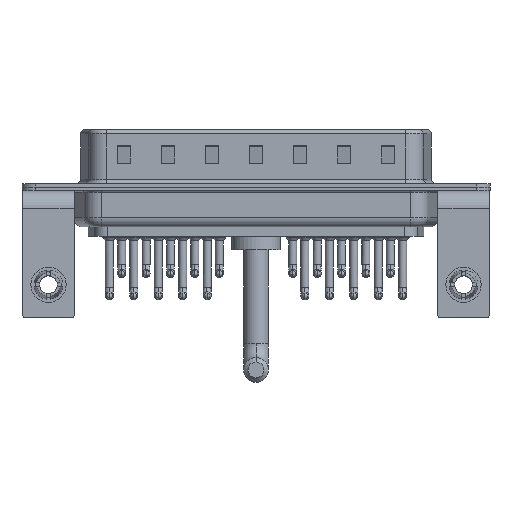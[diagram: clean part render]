
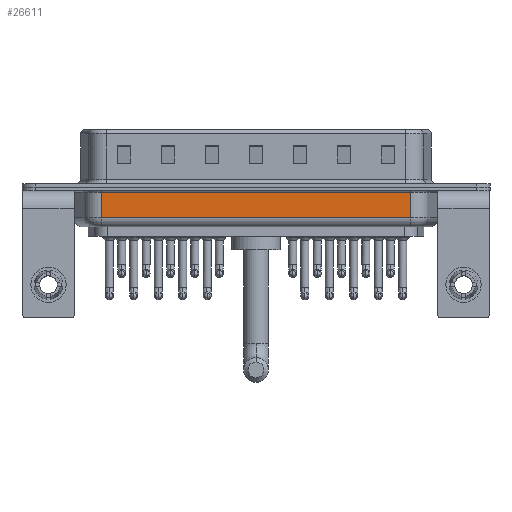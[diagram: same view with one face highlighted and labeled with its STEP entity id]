
A CAD part, front view. The second image highlights one B-rep face of the part: STEP entity #26611.
In plain terms, the highlighted planar face has unit normal (0, -1, 0).
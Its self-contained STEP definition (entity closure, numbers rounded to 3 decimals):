
#571 = DIRECTION ( 'NONE',  ( 0., 0., 1. ) ) ;
#2157 = VERTEX_POINT ( 'NONE', #11667 ) ;
#2365 = CARTESIAN_POINT ( 'NONE',  ( 6.006, -5.35, -3.5 ) ) ;
#2648 = CARTESIAN_POINT ( 'NONE',  ( 6.006, -5.35, -4.5 ) ) ;
#2704 = LINE ( 'NONE', #7304, #21092 ) ;
#2760 = ORIENTED_EDGE ( 'NONE', *, *, #17578, .T. ) ;
#3653 = EDGE_CURVE ( 'NONE', #2157, #20095, #26110, .T. ) ;
#4787 = ORIENTED_EDGE ( 'NONE', *, *, #15633, .T. ) ;
#4821 = FACE_OUTER_BOUND ( 'NONE', #18510, .T. ) ;
#4957 = DIRECTION ( 'NONE',  ( 0., 1., 0. ) ) ;
#5650 = CARTESIAN_POINT ( 'NONE',  ( 6.006, -5.35, -0.65 ) ) ;
#6526 = CARTESIAN_POINT ( 'NONE',  ( 41.044, -5.35, -4.5 ) ) ;
#7111 = PLANE ( 'NONE',  #12997 ) ;
#7304 = CARTESIAN_POINT ( 'NONE',  ( 6.006, -5.35, -4.5 ) ) ;
#8530 = LINE ( 'NONE', #2365, #20211 ) ;
#8814 = DIRECTION ( 'NONE',  ( 1., 0., 0. ) ) ;
#11242 = DIRECTION ( 'NONE',  ( 0., 0., 1. ) ) ;
#11667 = CARTESIAN_POINT ( 'NONE',  ( 41.044, -5.35, -3.5 ) ) ;
#12997 = AXIS2_PLACEMENT_3D ( 'NONE', #2648, #4957, #13672 ) ;
#13672 = DIRECTION ( 'NONE',  ( 0., 0., 1. ) ) ;
#13790 = CARTESIAN_POINT ( 'NONE',  ( 41.044, -5.35, -0.65 ) ) ;
#15633 = EDGE_CURVE ( 'NONE', #20095, #19097, #27819, .T. ) ;
#17578 = EDGE_CURVE ( 'NONE', #17929, #2157, #8530, .T. ) ;
#17929 = VERTEX_POINT ( 'NONE', #23518 ) ;
#18510 = EDGE_LOOP ( 'NONE', ( #27593, #2760, #25417, #4787 ) ) ;
#19097 = VERTEX_POINT ( 'NONE', #24629 ) ;
#19216 = VECTOR ( 'NONE', #11242, 1000. ) ;
#20095 = VERTEX_POINT ( 'NONE', #13790 ) ;
#20211 = VECTOR ( 'NONE', #8814, 1000. ) ;
#21092 = VECTOR ( 'NONE', #571, 1000. ) ;
#22233 = EDGE_CURVE ( 'NONE', #17929, #19097, #2704, .T. ) ;
#23518 = CARTESIAN_POINT ( 'NONE',  ( 6.006, -5.35, -3.5 ) ) ;
#24629 = CARTESIAN_POINT ( 'NONE',  ( 6.006, -5.35, -0.65 ) ) ;
#25417 = ORIENTED_EDGE ( 'NONE', *, *, #3653, .T. ) ;
#26110 = LINE ( 'NONE', #6526, #19216 ) ;
#26611 = ADVANCED_FACE ( 'NONE', ( #4821 ), #7111, .F. ) ;
#26961 = VECTOR ( 'NONE', #27401, 1000. ) ;
#27401 = DIRECTION ( 'NONE',  ( -1., 0., 0. ) ) ;
#27593 = ORIENTED_EDGE ( 'NONE', *, *, #22233, .F. ) ;
#27819 = LINE ( 'NONE', #5650, #26961 ) ;
